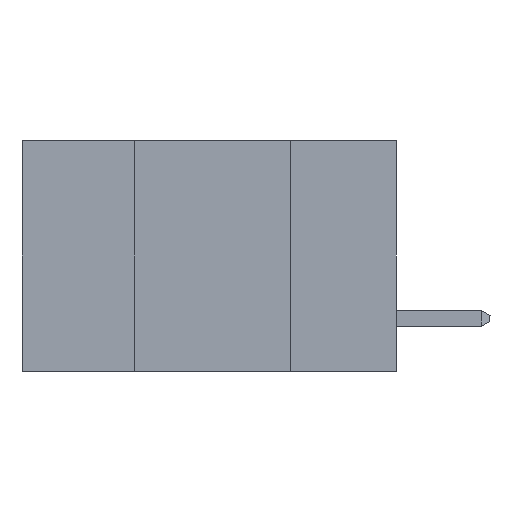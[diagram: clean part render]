
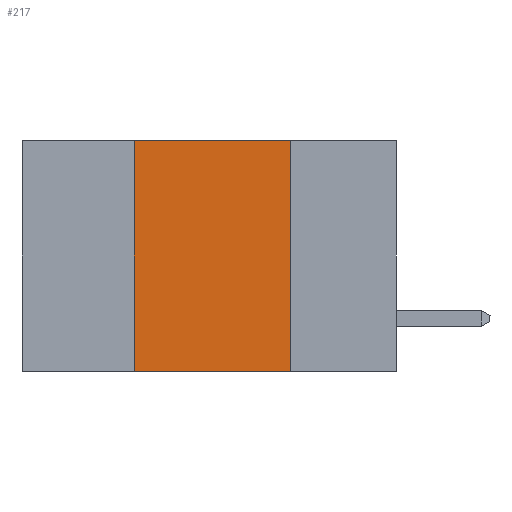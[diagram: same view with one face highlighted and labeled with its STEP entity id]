
A CAD part, left-side view. The second image highlights one B-rep face of the part: STEP entity #217.
In plain terms, the highlighted planar face has unit normal (-1, 0, 0).
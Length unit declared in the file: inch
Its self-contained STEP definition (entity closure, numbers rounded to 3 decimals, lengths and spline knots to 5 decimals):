
#217 = ADVANCED_FACE ( 'NONE', ( #1034 ), #7310, .F. ) ;
#809 = VERTEX_POINT ( 'NONE', #7625 ) ;
#886 = ORIENTED_EDGE ( 'NONE', *, *, #10762, .F. ) ;
#1034 = FACE_OUTER_BOUND ( 'NONE', #7617, .T. ) ;
#1275 = ORIENTED_EDGE ( 'NONE', *, *, #2585, .T. ) ;
#1403 = VERTEX_POINT ( 'NONE', #7285 ) ;
#1550 = CARTESIAN_POINT ( 'NONE',  ( 0., 0.6, -0.37 ) ) ;
#2386 = LINE ( 'NONE', #7088, #5221 ) ;
#2583 = VECTOR ( 'NONE', #10583, 39.37008 ) ;
#2585 = EDGE_CURVE ( 'NONE', #11022, #809, #5406, .T. ) ;
#3700 = DIRECTION ( 'NONE',  ( 0., 0., -1. ) ) ;
#4265 = LINE ( 'NONE', #4322, #6583 ) ;
#4322 = CARTESIAN_POINT ( 'NONE',  ( 0., 0.6, 0. ) ) ;
#4921 = VECTOR ( 'NONE', #3700, 39.37008 ) ;
#5221 = VECTOR ( 'NONE', #10833, 39.37008 ) ;
#5406 = LINE ( 'NONE', #1550, #2583 ) ;
#6363 = DIRECTION ( 'NONE',  ( 0., 0., -1. ) ) ;
#6387 = DIRECTION ( 'NONE',  ( 1., 0., 0. ) ) ;
#6446 = CARTESIAN_POINT ( 'NONE',  ( 0., 0.6, 0. ) ) ;
#6583 = VECTOR ( 'NONE', #11948, 39.37008 ) ;
#7088 = CARTESIAN_POINT ( 'NONE',  ( 0., 0.42, -0.37 ) ) ;
#7285 = CARTESIAN_POINT ( 'NONE',  ( 0., 0.17, 0. ) ) ;
#7310 = PLANE ( 'NONE',  #9368 ) ;
#7617 = EDGE_LOOP ( 'NONE', ( #10736, #12017, #886, #1275 ) ) ;
#7625 = CARTESIAN_POINT ( 'NONE',  ( 0., 0.17, -0.37 ) ) ;
#8240 = EDGE_CURVE ( 'NONE', #1403, #809, #9729, .T. ) ;
#9323 = CARTESIAN_POINT ( 'NONE',  ( 0., 0.42, -0.37 ) ) ;
#9368 = AXIS2_PLACEMENT_3D ( 'NONE', #6446, #6387, #6363 ) ;
#9542 = CARTESIAN_POINT ( 'NONE',  ( 0., 0.17, -0.37 ) ) ;
#9729 = LINE ( 'NONE', #9542, #4921 ) ;
#10150 = EDGE_CURVE ( 'NONE', #10889, #1403, #4265, .T. ) ;
#10583 = DIRECTION ( 'NONE',  ( 0., -1., 0. ) ) ;
#10736 = ORIENTED_EDGE ( 'NONE', *, *, #8240, .F. ) ;
#10762 = EDGE_CURVE ( 'NONE', #11022, #10889, #2386, .T. ) ;
#10833 = DIRECTION ( 'NONE',  ( 0., 0., 1. ) ) ;
#10889 = VERTEX_POINT ( 'NONE', #11040 ) ;
#11022 = VERTEX_POINT ( 'NONE', #9323 ) ;
#11040 = CARTESIAN_POINT ( 'NONE',  ( 0., 0.42, 0. ) ) ;
#11948 = DIRECTION ( 'NONE',  ( 0., -1., 0. ) ) ;
#12017 = ORIENTED_EDGE ( 'NONE', *, *, #10150, .F. ) ;
